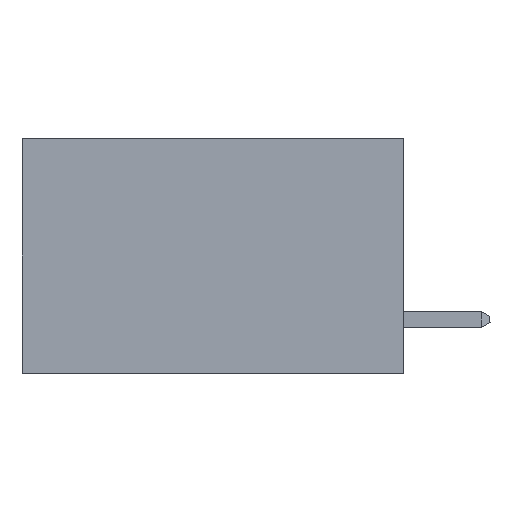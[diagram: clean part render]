
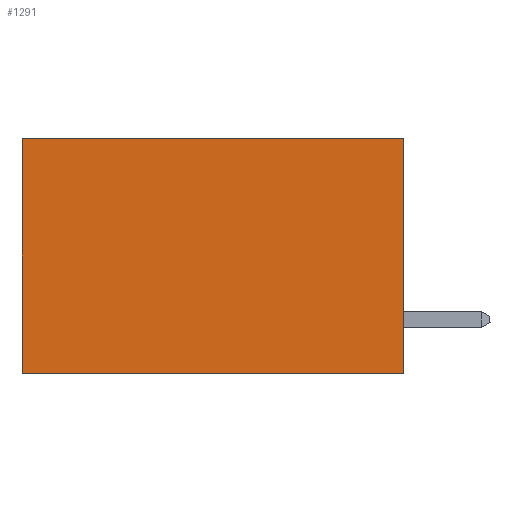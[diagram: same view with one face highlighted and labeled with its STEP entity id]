
A CAD part, left-side view. The second image highlights one B-rep face of the part: STEP entity #1291.
In plain terms, the highlighted planar face has unit normal (-1, 0, 0).
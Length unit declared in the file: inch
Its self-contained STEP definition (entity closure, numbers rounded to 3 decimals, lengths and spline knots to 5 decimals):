
#932 = LINE ( 'NONE', #19941, #15977 ) ;
#1291 = ADVANCED_FACE ( 'NONE', ( #16191 ), #9695, .F. ) ;
#2823 = LINE ( 'NONE', #20465, #12891 ) ;
#3658 = ORIENTED_EDGE ( 'NONE', *, *, #22961, .T. ) ;
#4010 = DIRECTION ( 'NONE',  ( 0., 1., 0. ) ) ;
#4357 = ORIENTED_EDGE ( 'NONE', *, *, #12422, .F. ) ;
#5258 = EDGE_CURVE ( 'NONE', #12231, #13960, #11245, .T. ) ;
#6074 = LINE ( 'NONE', #17113, #14831 ) ;
#6203 = VECTOR ( 'NONE', #12261, 39.37008 ) ;
#6311 = ORIENTED_EDGE ( 'NONE', *, *, #12039, .F. ) ;
#6835 = ORIENTED_EDGE ( 'NONE', *, *, #5258, .T. ) ;
#7997 = CARTESIAN_POINT ( 'NONE',  ( 0.2875, 0., 0. ) ) ;
#9695 = PLANE ( 'NONE',  #16689 ) ;
#11245 = LINE ( 'NONE', #19257, #6203 ) ;
#12039 = EDGE_CURVE ( 'NONE', #18903, #13960, #6074, .T. ) ;
#12177 = CARTESIAN_POINT ( 'NONE',  ( 0.2875, 0.6, 0. ) ) ;
#12231 = VERTEX_POINT ( 'NONE', #12177 ) ;
#12261 = DIRECTION ( 'NONE',  ( 0., 0., -1. ) ) ;
#12422 = EDGE_CURVE ( 'NONE', #15777, #18903, #932, .T. ) ;
#12459 = CARTESIAN_POINT ( 'NONE',  ( 0.2875, 0.6, -0.37 ) ) ;
#12891 = VECTOR ( 'NONE', #22209, 39.37008 ) ;
#13960 = VERTEX_POINT ( 'NONE', #12459 ) ;
#14831 = VECTOR ( 'NONE', #4010, 39.37008 ) ;
#14995 = CARTESIAN_POINT ( 'NONE',  ( 0.2875, 0., 0. ) ) ;
#15777 = VERTEX_POINT ( 'NONE', #7997 ) ;
#15977 = VECTOR ( 'NONE', #20019, 39.37008 ) ;
#16191 = FACE_OUTER_BOUND ( 'NONE', #22538, .T. ) ;
#16689 = AXIS2_PLACEMENT_3D ( 'NONE', #14995, #18699, #19717 ) ;
#17113 = CARTESIAN_POINT ( 'NONE',  ( 0.2875, 0., -0.37 ) ) ;
#18699 = DIRECTION ( 'NONE',  ( 1., 0., 0. ) ) ;
#18903 = VERTEX_POINT ( 'NONE', #22827 ) ;
#19257 = CARTESIAN_POINT ( 'NONE',  ( 0.2875, 0.6, 0. ) ) ;
#19717 = DIRECTION ( 'NONE',  ( 0., 0., -1. ) ) ;
#19941 = CARTESIAN_POINT ( 'NONE',  ( 0.2875, 0., 0. ) ) ;
#20019 = DIRECTION ( 'NONE',  ( 0., 0., -1. ) ) ;
#20465 = CARTESIAN_POINT ( 'NONE',  ( 0.2875, 0., 0. ) ) ;
#22209 = DIRECTION ( 'NONE',  ( 0., 1., 0. ) ) ;
#22538 = EDGE_LOOP ( 'NONE', ( #6835, #6311, #4357, #3658 ) ) ;
#22827 = CARTESIAN_POINT ( 'NONE',  ( 0.2875, 0., -0.37 ) ) ;
#22961 = EDGE_CURVE ( 'NONE', #15777, #12231, #2823, .T. ) ;
